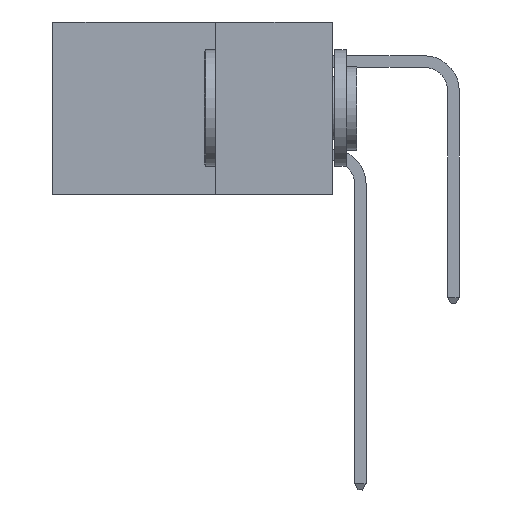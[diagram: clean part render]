
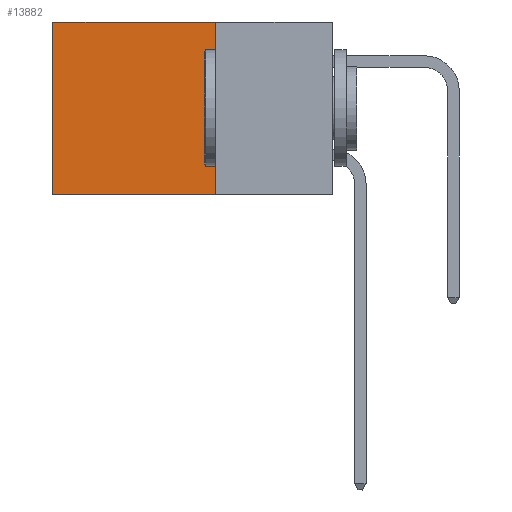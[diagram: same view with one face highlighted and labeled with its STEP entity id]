
A CAD part, left-side view. The second image highlights one B-rep face of the part: STEP entity #13882.
In plain terms, the highlighted planar face has unit normal (-1, 0, 0).
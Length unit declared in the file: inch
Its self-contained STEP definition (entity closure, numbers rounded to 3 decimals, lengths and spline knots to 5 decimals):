
#758 = DIRECTION ( 'NONE',  ( 1., 0., 0. ) ) ;
#2830 = EDGE_CURVE ( 'NONE', #8859, #4492, #18875, .T. ) ;
#2907 = DIRECTION ( 'NONE',  ( 0., 1., 0. ) ) ;
#3848 = CARTESIAN_POINT ( 'NONE',  ( 0.298, 0.25, -0.37 ) ) ;
#3883 = VECTOR ( 'NONE', #2907, 39.37008 ) ;
#4492 = VERTEX_POINT ( 'NONE', #4564 ) ;
#4564 = CARTESIAN_POINT ( 'NONE',  ( 0.298, 0.6, -0.37 ) ) ;
#4685 = LINE ( 'NONE', #16289, #8410 ) ;
#4957 = EDGE_CURVE ( 'NONE', #8500, #8859, #4685, .T. ) ;
#5651 = AXIS2_PLACEMENT_3D ( 'NONE', #16430, #758, #11894 ) ;
#8059 = CARTESIAN_POINT ( 'NONE',  ( 0.298, 0.25, -0.37 ) ) ;
#8109 = LINE ( 'NONE', #3848, #3883 ) ;
#8200 = EDGE_CURVE ( 'NONE', #8972, #4492, #8109, .T. ) ;
#8330 = ORIENTED_EDGE ( 'NONE', *, *, #8200, .F. ) ;
#8410 = VECTOR ( 'NONE', #12867, 39.37008 ) ;
#8500 = VERTEX_POINT ( 'NONE', #16933 ) ;
#8859 = VERTEX_POINT ( 'NONE', #9954 ) ;
#8972 = VERTEX_POINT ( 'NONE', #8059 ) ;
#9954 = CARTESIAN_POINT ( 'NONE',  ( 0.298, 0.6, 0. ) ) ;
#10980 = ORIENTED_EDGE ( 'NONE', *, *, #2830, .T. ) ;
#11772 = ORIENTED_EDGE ( 'NONE', *, *, #4957, .T. ) ;
#11894 = DIRECTION ( 'NONE',  ( 0., 0., -1. ) ) ;
#12384 = LINE ( 'NONE', #19529, #15959 ) ;
#12867 = DIRECTION ( 'NONE',  ( 0., 1., 0. ) ) ;
#13553 = FACE_OUTER_BOUND ( 'NONE', #16017, .T. ) ;
#13876 = ORIENTED_EDGE ( 'NONE', *, *, #14835, .F. ) ;
#13882 = ADVANCED_FACE ( 'NONE', ( #13553 ), #19437, .F. ) ;
#14835 = EDGE_CURVE ( 'NONE', #8500, #8972, #12384, .T. ) ;
#15027 = DIRECTION ( 'NONE',  ( 0., 0., -1. ) ) ;
#15959 = VECTOR ( 'NONE', #15027, 39.37008 ) ;
#16017 = EDGE_LOOP ( 'NONE', ( #10980, #8330, #13876, #11772 ) ) ;
#16289 = CARTESIAN_POINT ( 'NONE',  ( 0.298, 0.25, 0. ) ) ;
#16430 = CARTESIAN_POINT ( 'NONE',  ( 0.298, 0.25, 0. ) ) ;
#16673 = DIRECTION ( 'NONE',  ( 0., 0., -1. ) ) ;
#16680 = CARTESIAN_POINT ( 'NONE',  ( 0.298, 0.6, 0. ) ) ;
#16933 = CARTESIAN_POINT ( 'NONE',  ( 0.298, 0.25, 0. ) ) ;
#18406 = VECTOR ( 'NONE', #16673, 39.37008 ) ;
#18875 = LINE ( 'NONE', #16680, #18406 ) ;
#19437 = PLANE ( 'NONE',  #5651 ) ;
#19529 = CARTESIAN_POINT ( 'NONE',  ( 0.298, 0.25, 0. ) ) ;
